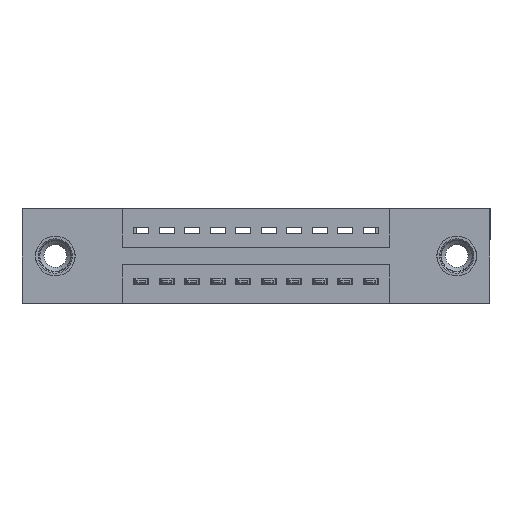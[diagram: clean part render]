
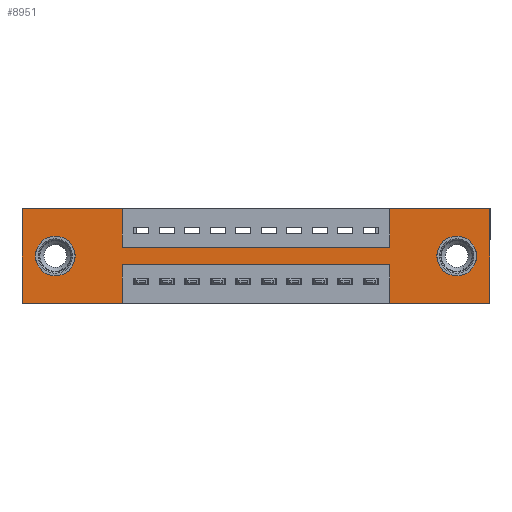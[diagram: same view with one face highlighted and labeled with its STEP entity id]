
A CAD part, front view. The second image highlights one B-rep face of the part: STEP entity #8951.
In plain terms, the highlighted planar face has unit normal (0, -1, 0).
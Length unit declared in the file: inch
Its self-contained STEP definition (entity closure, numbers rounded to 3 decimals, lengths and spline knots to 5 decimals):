
#63 = CARTESIAN_POINT ( 'NONE',  ( 0.3925, 0., -0.15 ) ) ;
#69 = CARTESIAN_POINT ( 'NONE',  ( 0.3925, 0., -0.22 ) ) ;
#114 = DIRECTION ( 'NONE',  ( 1., 0., 0. ) ) ;
#131 = DIRECTION ( 'NONE',  ( 0., 0., 1. ) ) ;
#383 = LINE ( 'NONE', #2519, #9391 ) ;
#442 = CIRCLE ( 'NONE', #2764, 0.078 ) ;
#524 = CARTESIAN_POINT ( 'NONE',  ( 0., 0., 0. ) ) ;
#588 = CARTESIAN_POINT ( 'NONE',  ( 1.4425, 0., -0.37 ) ) ;
#712 = DIRECTION ( 'NONE',  ( 0., 0., -1. ) ) ;
#978 = FACE_OUTER_BOUND ( 'NONE', #7821, .T. ) ;
#1104 = ORIENTED_EDGE ( 'NONE', *, *, #12444, .F. ) ;
#1279 = VERTEX_POINT ( 'NONE', #5288 ) ;
#1415 = VECTOR ( 'NONE', #9813, 39.37008 ) ;
#1660 = CARTESIAN_POINT ( 'NONE',  ( 1.4425, 0., -0.15 ) ) ;
#1801 = EDGE_CURVE ( 'NONE', #11066, #4272, #2444, .T. ) ;
#1956 = VECTOR ( 'NONE', #712, 39.37008 ) ;
#2129 = CARTESIAN_POINT ( 'NONE',  ( 1.4425, 0., -0.22 ) ) ;
#2175 = CARTESIAN_POINT ( 'NONE',  ( 0.13, 0., -0.185 ) ) ;
#2393 = CARTESIAN_POINT ( 'NONE',  ( 1.4425, 0., -0.37 ) ) ;
#2444 = LINE ( 'NONE', #4163, #4942 ) ;
#2501 = CARTESIAN_POINT ( 'NONE',  ( 1.4425, 0., 0. ) ) ;
#2519 = CARTESIAN_POINT ( 'NONE',  ( 0.3925, 0., -0.37 ) ) ;
#2587 = LINE ( 'NONE', #63, #4764 ) ;
#2591 = VERTEX_POINT ( 'NONE', #10302 ) ;
#2761 = CARTESIAN_POINT ( 'NONE',  ( 1.4425, 0., 0. ) ) ;
#2764 = AXIS2_PLACEMENT_3D ( 'NONE', #9055, #5035, #4808 ) ;
#2813 = CARTESIAN_POINT ( 'NONE',  ( 0.3925, 0., 0. ) ) ;
#2922 = DIRECTION ( 'NONE',  ( 0., 1., 0. ) ) ;
#2959 = ORIENTED_EDGE ( 'NONE', *, *, #10565, .F. ) ;
#3024 = EDGE_CURVE ( 'NONE', #2591, #9354, #9605, .T. ) ;
#3108 = EDGE_CURVE ( 'NONE', #4744, #1279, #11415, .T. ) ;
#3165 = LINE ( 'NONE', #588, #9684 ) ;
#3336 = EDGE_CURVE ( 'NONE', #6168, #4944, #6894, .T. ) ;
#3375 = EDGE_CURVE ( 'NONE', #4272, #9545, #11581, .T. ) ;
#3453 = LINE ( 'NONE', #2501, #9291 ) ;
#3578 = ORIENTED_EDGE ( 'NONE', *, *, #10591, .T. ) ;
#3771 = LINE ( 'NONE', #13644, #7226 ) ;
#3991 = EDGE_CURVE ( 'NONE', #4944, #8020, #383, .T. ) ;
#4095 = CIRCLE ( 'NONE', #5826, 0.078 ) ;
#4141 = DIRECTION ( 'NONE',  ( 0., 1., 0. ) ) ;
#4163 = CARTESIAN_POINT ( 'NONE',  ( 0., 0., 0. ) ) ;
#4270 = ORIENTED_EDGE ( 'NONE', *, *, #3375, .F. ) ;
#4272 = VERTEX_POINT ( 'NONE', #2813 ) ;
#4299 = LINE ( 'NONE', #8178, #1956 ) ;
#4326 = DIRECTION ( 'NONE',  ( 0., 0., 1. ) ) ;
#4368 = EDGE_CURVE ( 'NONE', #6676, #6391, #4095, .T. ) ;
#4414 = DIRECTION ( 'NONE',  ( 1., 0., 0. ) ) ;
#4744 = VERTEX_POINT ( 'NONE', #2761 ) ;
#4763 = DIRECTION ( 'NONE',  ( 0., 0., -1. ) ) ;
#4764 = VECTOR ( 'NONE', #114, 39.37008 ) ;
#4793 = ORIENTED_EDGE ( 'NONE', *, *, #10044, .F. ) ;
#4808 = DIRECTION ( 'NONE',  ( 0., 0., -1. ) ) ;
#4900 = EDGE_LOOP ( 'NONE', ( #13106, #13315 ) ) ;
#4942 = VECTOR ( 'NONE', #6282, 39.37008 ) ;
#4944 = VERTEX_POINT ( 'NONE', #8930 ) ;
#5035 = DIRECTION ( 'NONE',  ( 0., 1., 0. ) ) ;
#5193 = DIRECTION ( 'NONE',  ( 0., 0., -1. ) ) ;
#5288 = CARTESIAN_POINT ( 'NONE',  ( 1.835, 0., 0. ) ) ;
#5421 = ORIENTED_EDGE ( 'NONE', *, *, #13748, .F. ) ;
#5706 = DIRECTION ( 'NONE',  ( 0., 0., 1. ) ) ;
#5756 = DIRECTION ( 'NONE',  ( 0., 0., -1. ) ) ;
#5826 = AXIS2_PLACEMENT_3D ( 'NONE', #8459, #4141, #5193 ) ;
#5932 = EDGE_CURVE ( 'NONE', #9879, #11066, #7183, .T. ) ;
#6091 = DIRECTION ( 'NONE',  ( -1., 0., 0. ) ) ;
#6118 = VERTEX_POINT ( 'NONE', #2393 ) ;
#6168 = VERTEX_POINT ( 'NONE', #2129 ) ;
#6199 = ORIENTED_EDGE ( 'NONE', *, *, #3108, .F. ) ;
#6282 = DIRECTION ( 'NONE',  ( 1., 0., 0. ) ) ;
#6364 = CARTESIAN_POINT ( 'NONE',  ( 0., 0., -0.37 ) ) ;
#6391 = VERTEX_POINT ( 'NONE', #7137 ) ;
#6651 = VECTOR ( 'NONE', #9933, 39.37008 ) ;
#6676 = VERTEX_POINT ( 'NONE', #7698 ) ;
#6687 = AXIS2_PLACEMENT_3D ( 'NONE', #11512, #2922, #131 ) ;
#6881 = CARTESIAN_POINT ( 'NONE',  ( 0.3925, 0., -0.15 ) ) ;
#6894 = LINE ( 'NONE', #69, #1415 ) ;
#7137 = CARTESIAN_POINT ( 'NONE',  ( 1.705, 0., -0.263 ) ) ;
#7183 = LINE ( 'NONE', #524, #8185 ) ;
#7226 = VECTOR ( 'NONE', #6091, 39.37008 ) ;
#7698 = CARTESIAN_POINT ( 'NONE',  ( 1.705, 0., -0.107 ) ) ;
#7821 = EDGE_LOOP ( 'NONE', ( #11632, #10026, #8283, #1104, #9269, #6199, #5421, #4793, #4270, #12036, #11798, #2959 ) ) ;
#8003 = DIRECTION ( 'NONE',  ( 0., 0., 1. ) ) ;
#8020 = VERTEX_POINT ( 'NONE', #12636 ) ;
#8178 = CARTESIAN_POINT ( 'NONE',  ( 1.835, 0., 0. ) ) ;
#8185 = VECTOR ( 'NONE', #10139, 39.37008 ) ;
#8192 = ORIENTED_EDGE ( 'NONE', *, *, #3024, .T. ) ;
#8283 = ORIENTED_EDGE ( 'NONE', *, *, #8377, .F. ) ;
#8377 = EDGE_CURVE ( 'NONE', #6118, #6168, #3165, .T. ) ;
#8459 = CARTESIAN_POINT ( 'NONE',  ( 1.705, 0., -0.185 ) ) ;
#8828 = EDGE_LOOP ( 'NONE', ( #3578, #8192 ) ) ;
#8930 = CARTESIAN_POINT ( 'NONE',  ( 0.3925, 0., -0.22 ) ) ;
#8946 = CIRCLE ( 'NONE', #6687, 0.078 ) ;
#8951 = ADVANCED_FACE ( 'NONE', ( #11974, #9483, #978 ), #9156, .T. ) ;
#8985 = LINE ( 'NONE', #10939, #6651 ) ;
#9055 = CARTESIAN_POINT ( 'NONE',  ( 1.705, 0., -0.185 ) ) ;
#9122 = DIRECTION ( 'NONE',  ( 0., 0., -1. ) ) ;
#9156 = PLANE ( 'NONE',  #13472 ) ;
#9269 = ORIENTED_EDGE ( 'NONE', *, *, #13312, .F. ) ;
#9291 = VECTOR ( 'NONE', #5706, 39.37008 ) ;
#9354 = VERTEX_POINT ( 'NONE', #11773 ) ;
#9391 = VECTOR ( 'NONE', #4763, 39.37008 ) ;
#9483 = FACE_BOUND ( 'NONE', #8828, .T. ) ;
#9545 = VERTEX_POINT ( 'NONE', #6881 ) ;
#9605 = CIRCLE ( 'NONE', #13143, 0.078 ) ;
#9655 = EDGE_CURVE ( 'NONE', #6391, #6676, #442, .T. ) ;
#9684 = VECTOR ( 'NONE', #8003, 39.37008 ) ;
#9746 = CARTESIAN_POINT ( 'NONE',  ( 0., 0., 0. ) ) ;
#9813 = DIRECTION ( 'NONE',  ( -1., 0., 0. ) ) ;
#9879 = VERTEX_POINT ( 'NONE', #6364 ) ;
#9933 = DIRECTION ( 'NONE',  ( -1., 0., 0. ) ) ;
#10026 = ORIENTED_EDGE ( 'NONE', *, *, #3336, .F. ) ;
#10044 = EDGE_CURVE ( 'NONE', #9545, #11046, #2587, .T. ) ;
#10096 = VERTEX_POINT ( 'NONE', #11970 ) ;
#10139 = DIRECTION ( 'NONE',  ( 0., 0., 1. ) ) ;
#10302 = CARTESIAN_POINT ( 'NONE',  ( 0.13, 0., -0.263 ) ) ;
#10565 = EDGE_CURVE ( 'NONE', #8020, #9879, #3771, .T. ) ;
#10591 = EDGE_CURVE ( 'NONE', #9354, #2591, #8946, .T. ) ;
#10939 = CARTESIAN_POINT ( 'NONE',  ( 0., 0., -0.37 ) ) ;
#11046 = VERTEX_POINT ( 'NONE', #1660 ) ;
#11066 = VERTEX_POINT ( 'NONE', #11569 ) ;
#11208 = CARTESIAN_POINT ( 'NONE',  ( 0., 0., -0.37 ) ) ;
#11415 = LINE ( 'NONE', #9746, #13413 ) ;
#11512 = CARTESIAN_POINT ( 'NONE',  ( 0.13, 0., -0.185 ) ) ;
#11569 = CARTESIAN_POINT ( 'NONE',  ( 0., 0., 0. ) ) ;
#11581 = LINE ( 'NONE', #12153, #11911 ) ;
#11632 = ORIENTED_EDGE ( 'NONE', *, *, #3991, .F. ) ;
#11773 = CARTESIAN_POINT ( 'NONE',  ( 0.13, 0., -0.107 ) ) ;
#11798 = ORIENTED_EDGE ( 'NONE', *, *, #5932, .F. ) ;
#11911 = VECTOR ( 'NONE', #5756, 39.37008 ) ;
#11970 = CARTESIAN_POINT ( 'NONE',  ( 1.835, 0., -0.37 ) ) ;
#11974 = FACE_BOUND ( 'NONE', #4900, .T. ) ;
#12036 = ORIENTED_EDGE ( 'NONE', *, *, #1801, .F. ) ;
#12153 = CARTESIAN_POINT ( 'NONE',  ( 0.3925, 0., 0. ) ) ;
#12444 = EDGE_CURVE ( 'NONE', #10096, #6118, #8985, .T. ) ;
#12636 = CARTESIAN_POINT ( 'NONE',  ( 0.3925, 0., -0.37 ) ) ;
#12758 = DIRECTION ( 'NONE',  ( 0., -1., 0. ) ) ;
#12900 = DIRECTION ( 'NONE',  ( 0., 1., 0. ) ) ;
#13106 = ORIENTED_EDGE ( 'NONE', *, *, #4368, .T. ) ;
#13143 = AXIS2_PLACEMENT_3D ( 'NONE', #2175, #12900, #4326 ) ;
#13312 = EDGE_CURVE ( 'NONE', #1279, #10096, #4299, .T. ) ;
#13315 = ORIENTED_EDGE ( 'NONE', *, *, #9655, .T. ) ;
#13413 = VECTOR ( 'NONE', #4414, 39.37008 ) ;
#13472 = AXIS2_PLACEMENT_3D ( 'NONE', #11208, #12758, #9122 ) ;
#13644 = CARTESIAN_POINT ( 'NONE',  ( 0., 0., -0.37 ) ) ;
#13748 = EDGE_CURVE ( 'NONE', #11046, #4744, #3453, .T. ) ;
